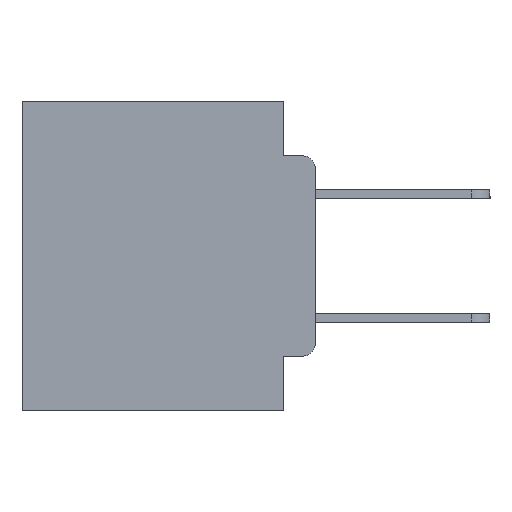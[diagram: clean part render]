
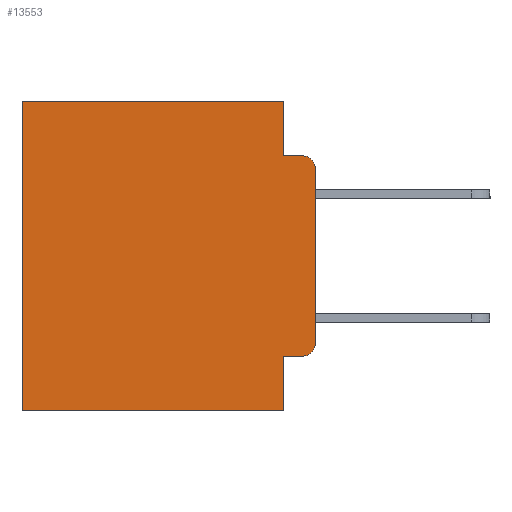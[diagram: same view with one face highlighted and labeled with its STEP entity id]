
A CAD part, left-side view. The second image highlights one B-rep face of the part: STEP entity #13553.
In plain terms, the highlighted planar face has unit normal (-1, 0, 0).
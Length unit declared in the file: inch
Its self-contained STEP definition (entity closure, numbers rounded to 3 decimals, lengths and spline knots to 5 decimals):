
#275 = VERTEX_POINT ( 'NONE', #10996 ) ;
#324 = VERTEX_POINT ( 'NONE', #17414 ) ;
#387 = DIRECTION ( 'NONE',  ( 0., 0., -1. ) ) ;
#631 = VERTEX_POINT ( 'NONE', #21574 ) ;
#650 = ORIENTED_EDGE ( 'NONE', *, *, #855, .F. ) ;
#655 = CARTESIAN_POINT ( 'NONE',  ( 0.298, 0.051, 0. ) ) ;
#855 = EDGE_CURVE ( 'NONE', #13434, #23593, #22685, .T. ) ;
#1253 = AXIS2_PLACEMENT_3D ( 'NONE', #17391, #17136, #387 ) ;
#2195 = ORIENTED_EDGE ( 'NONE', *, *, #23403, .T. ) ;
#2286 = VECTOR ( 'NONE', #17138, 39.37008 ) ;
#2440 = EDGE_CURVE ( 'NONE', #11757, #13434, #10177, .T. ) ;
#3371 = VERTEX_POINT ( 'NONE', #27921 ) ;
#3551 = VECTOR ( 'NONE', #9151, 39.37008 ) ;
#3558 = DIRECTION ( 'NONE',  ( 0., 0., -1. ) ) ;
#3789 = LINE ( 'NONE', #4225, #24751 ) ;
#4225 = CARTESIAN_POINT ( 'NONE',  ( 0.298, 0., -0.5 ) ) ;
#4885 = DIRECTION ( 'NONE',  ( 0., 0., -1. ) ) ;
#5314 = ORIENTED_EDGE ( 'NONE', *, *, #15119, .F. ) ;
#5386 = VERTEX_POINT ( 'NONE', #6630 ) ;
#5478 = EDGE_CURVE ( 'NONE', #24671, #3371, #21083, .T. ) ;
#5520 = EDGE_CURVE ( 'NONE', #275, #324, #25390, .T. ) ;
#5570 = LINE ( 'NONE', #24239, #10720 ) ;
#5735 = ORIENTED_EDGE ( 'NONE', *, *, #5520, .T. ) ;
#6630 = CARTESIAN_POINT ( 'NONE',  ( 0.298, 0., -0.1085 ) ) ;
#6929 = CARTESIAN_POINT ( 'NONE',  ( 0.298, 0., 0. ) ) ;
#7485 = CARTESIAN_POINT ( 'NONE',  ( 0.298, 0., 0. ) ) ;
#8010 = ORIENTED_EDGE ( 'NONE', *, *, #12872, .F. ) ;
#8096 = CARTESIAN_POINT ( 'NONE',  ( 0.298, 0.051, -0.0885 ) ) ;
#9151 = DIRECTION ( 'NONE',  ( 0., 1., 0. ) ) ;
#10142 = CARTESIAN_POINT ( 'NONE',  ( 0.298, 0., 0. ) ) ;
#10177 = LINE ( 'NONE', #19364, #15289 ) ;
#10720 = VECTOR ( 'NONE', #4885, 39.37008 ) ;
#10812 = AXIS2_PLACEMENT_3D ( 'NONE', #7485, #11914, #26797 ) ;
#10872 = CARTESIAN_POINT ( 'NONE',  ( 0.298, 0.473, 0. ) ) ;
#10996 = CARTESIAN_POINT ( 'NONE',  ( 0.298, 0.473, 0. ) ) ;
#11031 = FACE_OUTER_BOUND ( 'NONE', #11278, .T. ) ;
#11278 = EDGE_LOOP ( 'NONE', ( #24722, #2195, #650, #27673, #27073, #5735, #5314, #8010, #17237, #11532 ) ) ;
#11308 = VECTOR ( 'NONE', #14078, 39.37008 ) ;
#11412 = EDGE_CURVE ( 'NONE', #12666, #24671, #24218, .T. ) ;
#11532 = ORIENTED_EDGE ( 'NONE', *, *, #5478, .T. ) ;
#11757 = VERTEX_POINT ( 'NONE', #655 ) ;
#11914 = DIRECTION ( 'NONE',  ( 1., 0., 0. ) ) ;
#12593 = CARTESIAN_POINT ( 'NONE',  ( 0.298, 0.02, -0.1085 ) ) ;
#12666 = VERTEX_POINT ( 'NONE', #23487 ) ;
#12856 = VECTOR ( 'NONE', #23554, 39.37008 ) ;
#12872 = EDGE_CURVE ( 'NONE', #12666, #631, #5570, .T. ) ;
#13434 = VERTEX_POINT ( 'NONE', #20077 ) ;
#13553 = ADVANCED_FACE ( 'NONE', ( #11031 ), #16153, .F. ) ;
#14078 = DIRECTION ( 'NONE',  ( 0., -1., 0. ) ) ;
#14773 = DIRECTION ( 'NONE',  ( 0., 0., -1. ) ) ;
#15119 = EDGE_CURVE ( 'NONE', #631, #324, #3789, .T. ) ;
#15289 = VECTOR ( 'NONE', #18281, 39.37008 ) ;
#16153 = PLANE ( 'NONE',  #10812 ) ;
#17136 = DIRECTION ( 'NONE',  ( -1., 0., 0. ) ) ;
#17138 = DIRECTION ( 'NONE',  ( 0., 0., -1. ) ) ;
#17237 = ORIENTED_EDGE ( 'NONE', *, *, #11412, .T. ) ;
#17376 = DIRECTION ( 'NONE',  ( 0., 1., 0. ) ) ;
#17391 = CARTESIAN_POINT ( 'NONE',  ( 0.298, 0.02, -0.3915 ) ) ;
#17414 = CARTESIAN_POINT ( 'NONE',  ( 0.298, 0.473, -0.5 ) ) ;
#17493 = CARTESIAN_POINT ( 'NONE',  ( 0.298, 0.02, -0.0885 ) ) ;
#18281 = DIRECTION ( 'NONE',  ( 0., 0., -1. ) ) ;
#18856 = LINE ( 'NONE', #10142, #23834 ) ;
#19364 = CARTESIAN_POINT ( 'NONE',  ( 0.298, 0.051, 0. ) ) ;
#20077 = CARTESIAN_POINT ( 'NONE',  ( 0.298, 0.051, -0.0885 ) ) ;
#20585 = EDGE_CURVE ( 'NONE', #5386, #3371, #18856, .T. ) ;
#20882 = LINE ( 'NONE', #6929, #3551 ) ;
#21083 = CIRCLE ( 'NONE', #1253, 0.02 ) ;
#21431 = CARTESIAN_POINT ( 'NONE',  ( 0.298, 0.051, -0.4115 ) ) ;
#21574 = CARTESIAN_POINT ( 'NONE',  ( 0.298, 0.051, -0.5 ) ) ;
#22685 = LINE ( 'NONE', #8096, #11308 ) ;
#23403 = EDGE_CURVE ( 'NONE', #5386, #23593, #23704, .T. ) ;
#23452 = CARTESIAN_POINT ( 'NONE',  ( 0.298, 0.02, -0.4115 ) ) ;
#23487 = CARTESIAN_POINT ( 'NONE',  ( 0.298, 0.051, -0.4115 ) ) ;
#23554 = DIRECTION ( 'NONE',  ( 0., -1., 0. ) ) ;
#23593 = VERTEX_POINT ( 'NONE', #17493 ) ;
#23704 = CIRCLE ( 'NONE', #24285, 0.02 ) ;
#23834 = VECTOR ( 'NONE', #3558, 39.37008 ) ;
#24218 = LINE ( 'NONE', #21431, #12856 ) ;
#24239 = CARTESIAN_POINT ( 'NONE',  ( 0.298, 0.051, 0. ) ) ;
#24285 = AXIS2_PLACEMENT_3D ( 'NONE', #12593, #27449, #14773 ) ;
#24671 = VERTEX_POINT ( 'NONE', #23452 ) ;
#24722 = ORIENTED_EDGE ( 'NONE', *, *, #20585, .F. ) ;
#24751 = VECTOR ( 'NONE', #17376, 39.37008 ) ;
#25390 = LINE ( 'NONE', #10872, #2286 ) ;
#26155 = EDGE_CURVE ( 'NONE', #11757, #275, #20882, .T. ) ;
#26797 = DIRECTION ( 'NONE',  ( 0., 0., -1. ) ) ;
#27073 = ORIENTED_EDGE ( 'NONE', *, *, #26155, .T. ) ;
#27449 = DIRECTION ( 'NONE',  ( -1., 0., 0. ) ) ;
#27673 = ORIENTED_EDGE ( 'NONE', *, *, #2440, .F. ) ;
#27921 = CARTESIAN_POINT ( 'NONE',  ( 0.298, 0., -0.3915 ) ) ;
